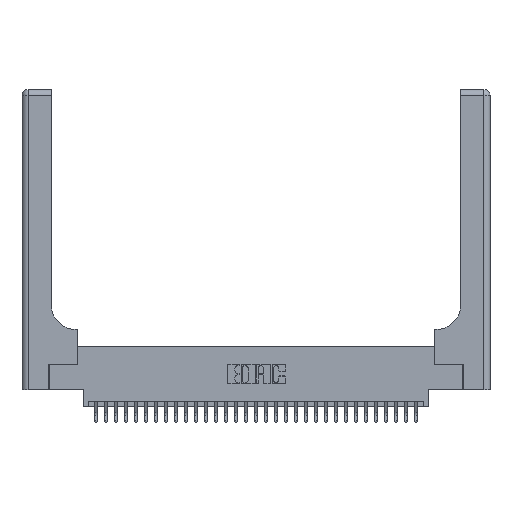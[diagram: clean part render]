
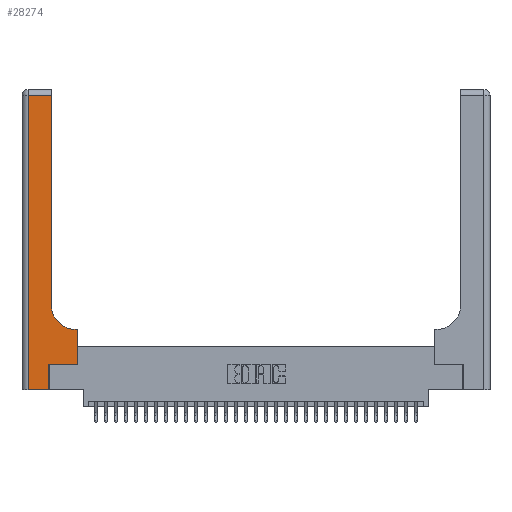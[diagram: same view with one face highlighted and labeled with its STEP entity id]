
A CAD part, top view. The second image highlights one B-rep face of the part: STEP entity #28274.
In plain terms, the highlighted planar face has unit normal (0, 0, 1).
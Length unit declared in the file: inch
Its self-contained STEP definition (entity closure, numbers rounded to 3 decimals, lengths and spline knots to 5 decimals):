
#16 = CARTESIAN_POINT ( 'NONE',  ( 0.269, 0., 0.37 ) ) ;
#647 = CARTESIAN_POINT ( 'NONE',  ( 0.5585, 0.6, 0.37 ) ) ;
#832 = EDGE_LOOP ( 'NONE', ( #18097, #13671, #22236, #18345, #28490, #10226, #1918, #22795, #25014 ) ) ;
#1035 = AXIS2_PLACEMENT_3D ( 'NONE', #21061, #23570, #16426 ) ;
#1302 = VERTEX_POINT ( 'NONE', #7041 ) ;
#1918 = ORIENTED_EDGE ( 'NONE', *, *, #9351, .T. ) ;
#1974 = VECTOR ( 'NONE', #14640, 39.37008 ) ;
#3757 = LINE ( 'NONE', #24229, #14864 ) ;
#4121 = CARTESIAN_POINT ( 'NONE',  ( 0.5585, 0.25, 0.37 ) ) ;
#4599 = DIRECTION ( 'NONE',  ( 0., 0., -1. ) ) ;
#4817 = DIRECTION ( 'NONE',  ( -1., 0., 0. ) ) ;
#6114 = VECTOR ( 'NONE', #8816, 39.37008 ) ;
#6355 = EDGE_CURVE ( 'NONE', #1302, #9731, #3757, .T. ) ;
#6645 = EDGE_CURVE ( 'NONE', #9959, #21293, #10464, .T. ) ;
#6765 = DIRECTION ( 'NONE',  ( 1., 0., 0. ) ) ;
#7041 = CARTESIAN_POINT ( 'NONE',  ( 0.06, 0., 0.37 ) ) ;
#7069 = CARTESIAN_POINT ( 'NONE',  ( 0.2915, 0.85, 0.37 ) ) ;
#7178 = CARTESIAN_POINT ( 'NONE',  ( 0.269, 0.25, 0.37 ) ) ;
#7196 = VERTEX_POINT ( 'NONE', #647 ) ;
#7821 = CARTESIAN_POINT ( 'NONE',  ( 0.269, 0., 0.37 ) ) ;
#8773 = EDGE_CURVE ( 'NONE', #21293, #18148, #10826, .T. ) ;
#8816 = DIRECTION ( 'NONE',  ( 0., 1., 0. ) ) ;
#9351 = EDGE_CURVE ( 'NONE', #22075, #7196, #26181, .T. ) ;
#9731 = VERTEX_POINT ( 'NONE', #7821 ) ;
#9801 = DIRECTION ( 'NONE',  ( -1., 0., 0. ) ) ;
#9915 = PLANE ( 'NONE',  #29990 ) ;
#9959 = VERTEX_POINT ( 'NONE', #7069 ) ;
#10226 = ORIENTED_EDGE ( 'NONE', *, *, #10864, .T. ) ;
#10464 = LINE ( 'NONE', #24857, #6114 ) ;
#10826 = LINE ( 'NONE', #15124, #29752 ) ;
#10864 = EDGE_CURVE ( 'NONE', #13268, #22075, #23727, .T. ) ;
#12818 = EDGE_CURVE ( 'NONE', #9731, #13268, #14973, .T. ) ;
#13268 = VERTEX_POINT ( 'NONE', #17168 ) ;
#13671 = ORIENTED_EDGE ( 'NONE', *, *, #8773, .T. ) ;
#14640 = DIRECTION ( 'NONE',  ( -1., 0., 0. ) ) ;
#14745 = CARTESIAN_POINT ( 'NONE',  ( 0.2915, 0.6, 0.37 ) ) ;
#14864 = VECTOR ( 'NONE', #6765, 39.37008 ) ;
#14973 = LINE ( 'NONE', #16, #20889 ) ;
#15124 = CARTESIAN_POINT ( 'NONE',  ( 0., 2.94, 0.37 ) ) ;
#15833 = LINE ( 'NONE', #14745, #1974 ) ;
#16115 = EDGE_CURVE ( 'NONE', #7196, #22597, #15833, .T. ) ;
#16426 = DIRECTION ( 'NONE',  ( 1., 0., 0. ) ) ;
#17168 = CARTESIAN_POINT ( 'NONE',  ( 0.269, 0.25, 0.37 ) ) ;
#18097 = ORIENTED_EDGE ( 'NONE', *, *, #6645, .T. ) ;
#18148 = VERTEX_POINT ( 'NONE', #25562 ) ;
#18345 = ORIENTED_EDGE ( 'NONE', *, *, #6355, .T. ) ;
#18484 = CIRCLE ( 'NONE', #1035, 0.25 ) ;
#18878 = VECTOR ( 'NONE', #21985, 39.37008 ) ;
#19354 = FACE_OUTER_BOUND ( 'NONE', #832, .T. ) ;
#19424 = DIRECTION ( 'NONE',  ( 0., 1., 0. ) ) ;
#20889 = VECTOR ( 'NONE', #22585, 39.37008 ) ;
#21061 = CARTESIAN_POINT ( 'NONE',  ( 0.5415, 0.85, 0.37 ) ) ;
#21293 = VERTEX_POINT ( 'NONE', #23900 ) ;
#21985 = DIRECTION ( 'NONE',  ( 0., -1., 0. ) ) ;
#22075 = VERTEX_POINT ( 'NONE', #29672 ) ;
#22091 = CARTESIAN_POINT ( 'NONE',  ( 0.5415, 0.6, 0.37 ) ) ;
#22097 = CARTESIAN_POINT ( 'NONE',  ( 0.06, 3., 0.37 ) ) ;
#22236 = ORIENTED_EDGE ( 'NONE', *, *, #26304, .T. ) ;
#22585 = DIRECTION ( 'NONE',  ( 0., 1., 0. ) ) ;
#22597 = VERTEX_POINT ( 'NONE', #22091 ) ;
#22795 = ORIENTED_EDGE ( 'NONE', *, *, #16115, .T. ) ;
#23570 = DIRECTION ( 'NONE',  ( 0., 0., -1. ) ) ;
#23727 = LINE ( 'NONE', #7178, #31179 ) ;
#23900 = CARTESIAN_POINT ( 'NONE',  ( 0.2915, 2.94, 0.37 ) ) ;
#24229 = CARTESIAN_POINT ( 'NONE',  ( 0., 0., 0.37 ) ) ;
#24857 = CARTESIAN_POINT ( 'NONE',  ( 0.2915, 3., 0.37 ) ) ;
#24871 = DIRECTION ( 'NONE',  ( 1., 0., 0. ) ) ;
#25014 = ORIENTED_EDGE ( 'NONE', *, *, #29299, .T. ) ;
#25562 = CARTESIAN_POINT ( 'NONE',  ( 0.06, 2.94, 0.37 ) ) ;
#26181 = LINE ( 'NONE', #4121, #30503 ) ;
#26304 = EDGE_CURVE ( 'NONE', #18148, #1302, #31051, .T. ) ;
#28274 = ADVANCED_FACE ( 'NONE', ( #19354 ), #9915, .F. ) ;
#28490 = ORIENTED_EDGE ( 'NONE', *, *, #12818, .T. ) ;
#29299 = EDGE_CURVE ( 'NONE', #22597, #9959, #18484, .T. ) ;
#29672 = CARTESIAN_POINT ( 'NONE',  ( 0.5585, 0.25, 0.37 ) ) ;
#29739 = CARTESIAN_POINT ( 'NONE',  ( 0., 3., 0.37 ) ) ;
#29752 = VECTOR ( 'NONE', #4817, 39.37008 ) ;
#29990 = AXIS2_PLACEMENT_3D ( 'NONE', #29739, #4599, #9801 ) ;
#30503 = VECTOR ( 'NONE', #19424, 39.37008 ) ;
#31051 = LINE ( 'NONE', #22097, #18878 ) ;
#31179 = VECTOR ( 'NONE', #24871, 39.37008 ) ;
